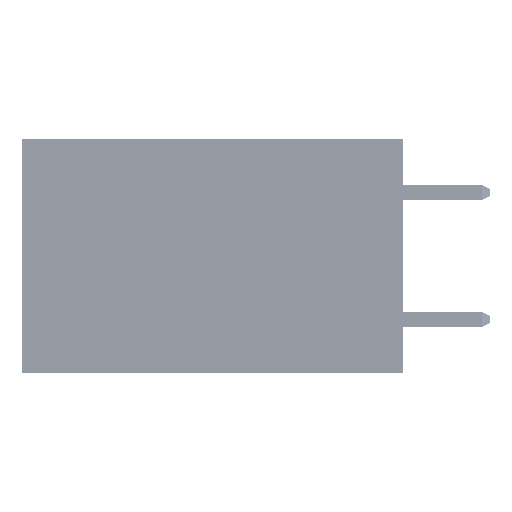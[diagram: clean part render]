
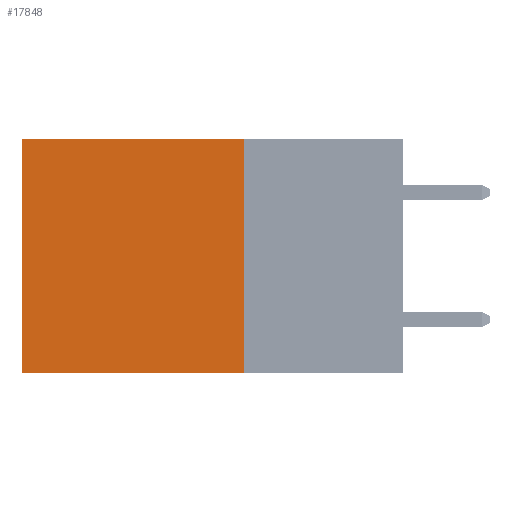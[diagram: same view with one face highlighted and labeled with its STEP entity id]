
A CAD part, left-side view. The second image highlights one B-rep face of the part: STEP entity #17848.
In plain terms, the highlighted planar face has unit normal (-1, 0, 0).
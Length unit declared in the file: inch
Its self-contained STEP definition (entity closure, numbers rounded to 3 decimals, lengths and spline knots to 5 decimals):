
#88 = VECTOR ( 'NONE', #4122, 39.37008 ) ;
#2543 = LINE ( 'NONE', #22049, #43364 ) ;
#2579 = EDGE_CURVE ( 'NONE', #47921, #16013, #36546, .T. ) ;
#2610 = DIRECTION ( 'NONE',  ( 1., 0., 0. ) ) ;
#2946 = DIRECTION ( 'NONE',  ( 0., 0., -1. ) ) ;
#4122 = DIRECTION ( 'NONE',  ( 0., 0., -1. ) ) ;
#9545 = LINE ( 'NONE', #28045, #28740 ) ;
#10044 = DIRECTION ( 'NONE',  ( 0., 1., 0. ) ) ;
#10173 = VERTEX_POINT ( 'NONE', #13804 ) ;
#10593 = VECTOR ( 'NONE', #10044, 39.37008 ) ;
#10860 = EDGE_CURVE ( 'NONE', #38931, #10173, #2543, .T. ) ;
#12126 = DIRECTION ( 'NONE',  ( 0., 0., -1. ) ) ;
#13804 = CARTESIAN_POINT ( 'NONE',  ( 0.2875, 0.6, -0.37 ) ) ;
#15023 = ORIENTED_EDGE ( 'NONE', *, *, #18755, .F. ) ;
#15546 = CARTESIAN_POINT ( 'NONE',  ( 0.2875, 0.25, 0. ) ) ;
#16013 = VERTEX_POINT ( 'NONE', #38086 ) ;
#17848 = ADVANCED_FACE ( 'NONE', ( #50013 ), #46325, .F. ) ;
#18755 = EDGE_CURVE ( 'NONE', #47921, #38931, #9545, .T. ) ;
#19865 = LINE ( 'NONE', #39914, #88 ) ;
#21544 = DIRECTION ( 'NONE',  ( 0., 1., 0. ) ) ;
#22049 = CARTESIAN_POINT ( 'NONE',  ( 0.2875, 0.25, -0.37 ) ) ;
#24613 = ORIENTED_EDGE ( 'NONE', *, *, #10860, .F. ) ;
#28045 = CARTESIAN_POINT ( 'NONE',  ( 0.2875, 0.25, 0. ) ) ;
#28740 = VECTOR ( 'NONE', #12126, 39.37008 ) ;
#29913 = CARTESIAN_POINT ( 'NONE',  ( 0.2875, 0.25, 0. ) ) ;
#31846 = EDGE_CURVE ( 'NONE', #16013, #10173, #19865, .T. ) ;
#33352 = ORIENTED_EDGE ( 'NONE', *, *, #31846, .T. ) ;
#34085 = ORIENTED_EDGE ( 'NONE', *, *, #2579, .T. ) ;
#36546 = LINE ( 'NONE', #29913, #10593 ) ;
#38086 = CARTESIAN_POINT ( 'NONE',  ( 0.2875, 0.6, 0. ) ) ;
#38216 = CARTESIAN_POINT ( 'NONE',  ( 0.2875, 0.25, 0. ) ) ;
#38914 = EDGE_LOOP ( 'NONE', ( #33352, #24613, #15023, #34085 ) ) ;
#38931 = VERTEX_POINT ( 'NONE', #38983 ) ;
#38983 = CARTESIAN_POINT ( 'NONE',  ( 0.2875, 0.25, -0.37 ) ) ;
#39914 = CARTESIAN_POINT ( 'NONE',  ( 0.2875, 0.6, 0. ) ) ;
#43364 = VECTOR ( 'NONE', #21544, 39.37008 ) ;
#43944 = AXIS2_PLACEMENT_3D ( 'NONE', #38216, #2610, #2946 ) ;
#46325 = PLANE ( 'NONE',  #43944 ) ;
#47921 = VERTEX_POINT ( 'NONE', #15546 ) ;
#50013 = FACE_OUTER_BOUND ( 'NONE', #38914, .T. ) ;
